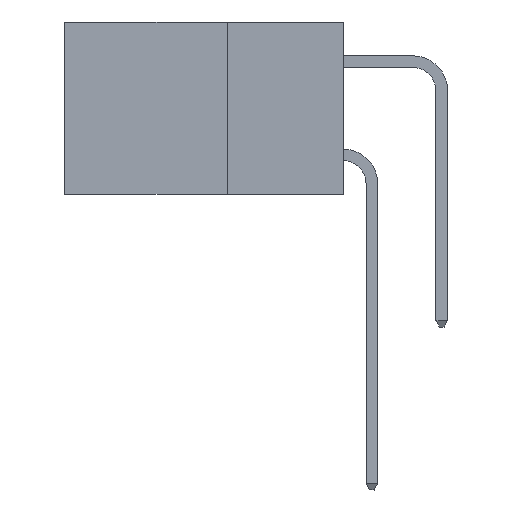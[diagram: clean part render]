
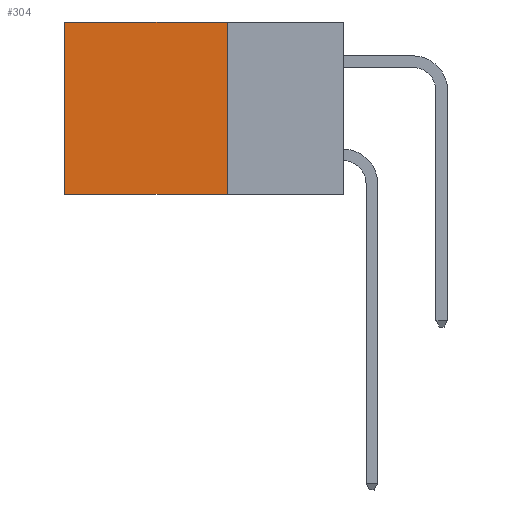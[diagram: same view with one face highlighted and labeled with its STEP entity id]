
A CAD part, left-side view. The second image highlights one B-rep face of the part: STEP entity #304.
In plain terms, the highlighted planar face has unit normal (-1, 0, 0).
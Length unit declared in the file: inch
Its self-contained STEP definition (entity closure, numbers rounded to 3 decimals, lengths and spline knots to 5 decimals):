
#236 = ORIENTED_EDGE ( 'NONE', *, *, #8619, .F. ) ;
#304 = ADVANCED_FACE ( 'NONE', ( #2034 ), #6702, .F. ) ;
#384 = DIRECTION ( 'NONE',  ( 0., 0., -1. ) ) ;
#535 = ORIENTED_EDGE ( 'NONE', *, *, #6848, .T. ) ;
#602 = ORIENTED_EDGE ( 'NONE', *, *, #3496, .T. ) ;
#1144 = VERTEX_POINT ( 'NONE', #3192 ) ;
#1298 = LINE ( 'NONE', #5727, #3571 ) ;
#1606 = EDGE_LOOP ( 'NONE', ( #535, #5101, #236, #602 ) ) ;
#2034 = FACE_OUTER_BOUND ( 'NONE', #1606, .T. ) ;
#2062 = LINE ( 'NONE', #9594, #6754 ) ;
#2271 = VERTEX_POINT ( 'NONE', #5036 ) ;
#3192 = CARTESIAN_POINT ( 'NONE',  ( 0.298, 0.25, -0.37 ) ) ;
#3381 = DIRECTION ( 'NONE',  ( 0., 1., 0. ) ) ;
#3496 = EDGE_CURVE ( 'NONE', #5498, #4624, #7948, .T. ) ;
#3571 = VECTOR ( 'NONE', #9204, 39.37008 ) ;
#4624 = VERTEX_POINT ( 'NONE', #7636 ) ;
#4700 = AXIS2_PLACEMENT_3D ( 'NONE', #7789, #5517, #384 ) ;
#4993 = VECTOR ( 'NONE', #9764, 39.37008 ) ;
#5036 = CARTESIAN_POINT ( 'NONE',  ( 0.298, 0.6, -0.37 ) ) ;
#5101 = ORIENTED_EDGE ( 'NONE', *, *, #11522, .F. ) ;
#5365 = CARTESIAN_POINT ( 'NONE',  ( 0.298, 0.25, 0. ) ) ;
#5498 = VERTEX_POINT ( 'NONE', #10180 ) ;
#5517 = DIRECTION ( 'NONE',  ( 1., 0., 0. ) ) ;
#5580 = LINE ( 'NONE', #5365, #4993 ) ;
#5727 = CARTESIAN_POINT ( 'NONE',  ( 0.298, 0.6, 0. ) ) ;
#6533 = DIRECTION ( 'NONE',  ( 0., 1., 0. ) ) ;
#6690 = CARTESIAN_POINT ( 'NONE',  ( 0.298, 0.25, 0. ) ) ;
#6702 = PLANE ( 'NONE',  #4700 ) ;
#6754 = VECTOR ( 'NONE', #3381, 39.37008 ) ;
#6848 = EDGE_CURVE ( 'NONE', #4624, #2271, #1298, .T. ) ;
#7636 = CARTESIAN_POINT ( 'NONE',  ( 0.298, 0.6, 0. ) ) ;
#7644 = VECTOR ( 'NONE', #6533, 39.37008 ) ;
#7789 = CARTESIAN_POINT ( 'NONE',  ( 0.298, 0.25, 0. ) ) ;
#7948 = LINE ( 'NONE', #6690, #7644 ) ;
#8619 = EDGE_CURVE ( 'NONE', #5498, #1144, #5580, .T. ) ;
#9204 = DIRECTION ( 'NONE',  ( 0., 0., -1. ) ) ;
#9594 = CARTESIAN_POINT ( 'NONE',  ( 0.298, 0.25, -0.37 ) ) ;
#9764 = DIRECTION ( 'NONE',  ( 0., 0., -1. ) ) ;
#10180 = CARTESIAN_POINT ( 'NONE',  ( 0.298, 0.25, 0. ) ) ;
#11522 = EDGE_CURVE ( 'NONE', #1144, #2271, #2062, .T. ) ;
